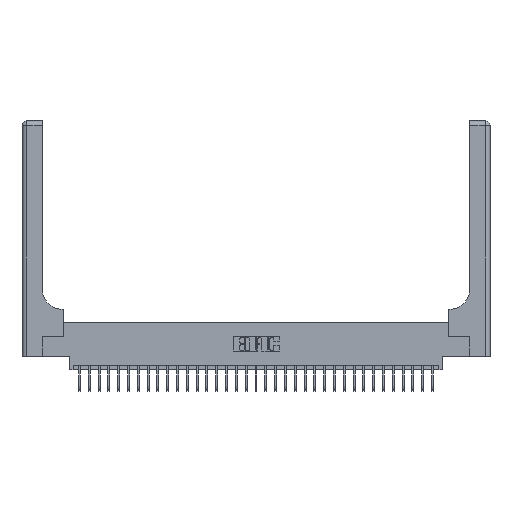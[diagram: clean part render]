
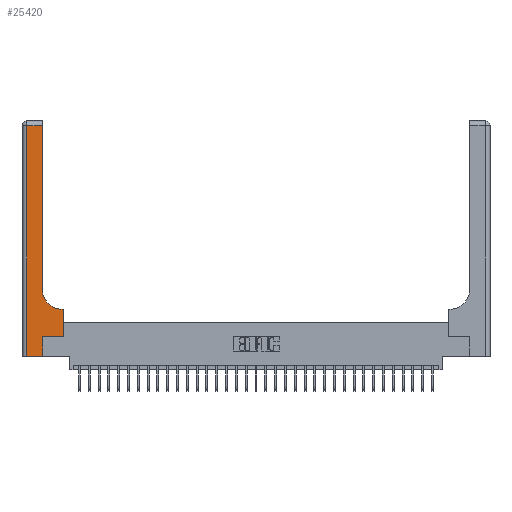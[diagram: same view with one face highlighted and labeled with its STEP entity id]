
A CAD part, top view. The second image highlights one B-rep face of the part: STEP entity #25420.
In plain terms, the highlighted planar face has unit normal (0, 0, 1).
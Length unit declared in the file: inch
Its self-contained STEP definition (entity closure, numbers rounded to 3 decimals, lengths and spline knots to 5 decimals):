
#75 = VECTOR ( 'NONE', #26460, 39.37008 ) ;
#302 = DIRECTION ( 'NONE',  ( 1., 0., 0. ) ) ;
#389 = DIRECTION ( 'NONE',  ( -1., 0., 0. ) ) ;
#628 = CARTESIAN_POINT ( 'NONE',  ( 0., 0., 0.37 ) ) ;
#992 = VERTEX_POINT ( 'NONE', #19337 ) ;
#1406 = DIRECTION ( 'NONE',  ( 0., 1., 0. ) ) ;
#1506 = ORIENTED_EDGE ( 'NONE', *, *, #29371, .T. ) ;
#1662 = ORIENTED_EDGE ( 'NONE', *, *, #29069, .T. ) ;
#1669 = DIRECTION ( 'NONE',  ( 0., 1., 0. ) ) ;
#3080 = VECTOR ( 'NONE', #3709, 39.37008 ) ;
#3547 = CARTESIAN_POINT ( 'NONE',  ( 0.26, 2.94, 0.37 ) ) ;
#3709 = DIRECTION ( 'NONE',  ( 0., -1., 0. ) ) ;
#3958 = ORIENTED_EDGE ( 'NONE', *, *, #13010, .T. ) ;
#4423 = VERTEX_POINT ( 'NONE', #10395 ) ;
#5325 = VECTOR ( 'NONE', #1406, 39.37008 ) ;
#6038 = DIRECTION ( 'NONE',  ( 0., 0., -1. ) ) ;
#6197 = CARTESIAN_POINT ( 'NONE',  ( 0.265, 0.25, 0.37 ) ) ;
#6236 = VERTEX_POINT ( 'NONE', #10436 ) ;
#6253 = ORIENTED_EDGE ( 'NONE', *, *, #24538, .T. ) ;
#6931 = VERTEX_POINT ( 'NONE', #20930 ) ;
#7708 = ORIENTED_EDGE ( 'NONE', *, *, #10326, .T. ) ;
#8178 = CARTESIAN_POINT ( 'NONE',  ( 0.528, 0.25, 0.37 ) ) ;
#8243 = LINE ( 'NONE', #14781, #20572 ) ;
#8469 = ORIENTED_EDGE ( 'NONE', *, *, #16664, .T. ) ;
#8545 = DIRECTION ( 'NONE',  ( 0., 0., -1. ) ) ;
#9195 = EDGE_CURVE ( 'NONE', #6931, #6236, #27051, .T. ) ;
#9404 = LINE ( 'NONE', #25782, #23468 ) ;
#9490 = ORIENTED_EDGE ( 'NONE', *, *, #19583, .T. ) ;
#9709 = LINE ( 'NONE', #8178, #5325 ) ;
#10071 = CARTESIAN_POINT ( 'NONE',  ( 0.06, 0., 0.37 ) ) ;
#10128 = CARTESIAN_POINT ( 'NONE',  ( 0., 3., 0.37 ) ) ;
#10326 = EDGE_CURVE ( 'NONE', #6236, #16020, #9709, .T. ) ;
#10395 = CARTESIAN_POINT ( 'NONE',  ( 0.51, 0.6, 0.37 ) ) ;
#10436 = CARTESIAN_POINT ( 'NONE',  ( 0.528, 0.25, 0.37 ) ) ;
#10768 = CIRCLE ( 'NONE', #26913, 0.25 ) ;
#10778 = VERTEX_POINT ( 'NONE', #10071 ) ;
#11673 = CARTESIAN_POINT ( 'NONE',  ( 0.06, 2.94, 0.37 ) ) ;
#12179 = DIRECTION ( 'NONE',  ( -1., 0., 0. ) ) ;
#12787 = AXIS2_PLACEMENT_3D ( 'NONE', #10128, #6038, #12179 ) ;
#13010 = EDGE_CURVE ( 'NONE', #16020, #4423, #20177, .T. ) ;
#13670 = EDGE_LOOP ( 'NONE', ( #8469, #1506, #19479, #6253, #1662, #16209, #7708, #3958, #9490 ) ) ;
#14781 = CARTESIAN_POINT ( 'NONE',  ( 0.265, 0., 0.37 ) ) ;
#15133 = PLANE ( 'NONE',  #12787 ) ;
#15377 = LINE ( 'NONE', #26851, #3080 ) ;
#16020 = VERTEX_POINT ( 'NONE', #23218 ) ;
#16209 = ORIENTED_EDGE ( 'NONE', *, *, #9195, .T. ) ;
#16664 = EDGE_CURVE ( 'NONE', #992, #26182, #21968, .T. ) ;
#17211 = CARTESIAN_POINT ( 'NONE',  ( 0.26, 0.6, 0.37 ) ) ;
#17304 = DIRECTION ( 'NONE',  ( 0., 1., 0. ) ) ;
#19337 = CARTESIAN_POINT ( 'NONE',  ( 0.26, 0.85, 0.37 ) ) ;
#19479 = ORIENTED_EDGE ( 'NONE', *, *, #19673, .T. ) ;
#19583 = EDGE_CURVE ( 'NONE', #4423, #992, #10768, .T. ) ;
#19673 = EDGE_CURVE ( 'NONE', #25694, #10778, #15377, .T. ) ;
#19750 = DIRECTION ( 'NONE',  ( 1., 0., 0. ) ) ;
#20177 = LINE ( 'NONE', #17211, #75 ) ;
#20572 = VECTOR ( 'NONE', #17304, 39.37008 ) ;
#20930 = CARTESIAN_POINT ( 'NONE',  ( 0.265, 0.25, 0.37 ) ) ;
#21102 = CARTESIAN_POINT ( 'NONE',  ( 0.265, 0., 0.37 ) ) ;
#21674 = CARTESIAN_POINT ( 'NONE',  ( 0.26, 3., 0.37 ) ) ;
#21968 = LINE ( 'NONE', #21674, #26587 ) ;
#22371 = VECTOR ( 'NONE', #19750, 39.37008 ) ;
#22713 = VERTEX_POINT ( 'NONE', #21102 ) ;
#23218 = CARTESIAN_POINT ( 'NONE',  ( 0.528, 0.6, 0.37 ) ) ;
#23468 = VECTOR ( 'NONE', #389, 39.37008 ) ;
#24480 = DIRECTION ( 'NONE',  ( 1., 0., 0. ) ) ;
#24538 = EDGE_CURVE ( 'NONE', #10778, #22713, #25692, .T. ) ;
#24752 = VECTOR ( 'NONE', #302, 39.37008 ) ;
#25420 = ADVANCED_FACE ( 'NONE', ( #26476 ), #15133, .F. ) ;
#25692 = LINE ( 'NONE', #628, #24752 ) ;
#25694 = VERTEX_POINT ( 'NONE', #11673 ) ;
#25782 = CARTESIAN_POINT ( 'NONE',  ( 0., 2.94, 0.37 ) ) ;
#26182 = VERTEX_POINT ( 'NONE', #3547 ) ;
#26460 = DIRECTION ( 'NONE',  ( -1., 0., 0. ) ) ;
#26476 = FACE_OUTER_BOUND ( 'NONE', #13670, .T. ) ;
#26587 = VECTOR ( 'NONE', #1669, 39.37008 ) ;
#26708 = CARTESIAN_POINT ( 'NONE',  ( 0.51, 0.85, 0.37 ) ) ;
#26851 = CARTESIAN_POINT ( 'NONE',  ( 0.06, 3., 0.37 ) ) ;
#26913 = AXIS2_PLACEMENT_3D ( 'NONE', #26708, #8545, #24480 ) ;
#27051 = LINE ( 'NONE', #6197, #22371 ) ;
#29069 = EDGE_CURVE ( 'NONE', #22713, #6931, #8243, .T. ) ;
#29371 = EDGE_CURVE ( 'NONE', #26182, #25694, #9404, .T. ) ;
